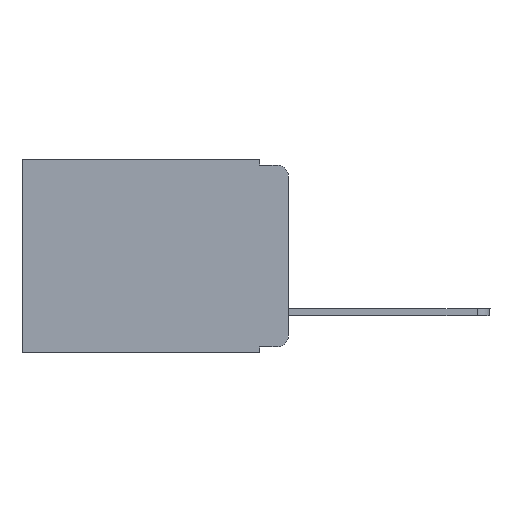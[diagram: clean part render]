
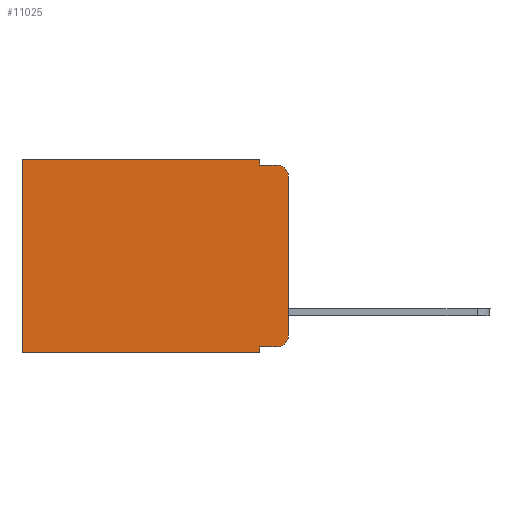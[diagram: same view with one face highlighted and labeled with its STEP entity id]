
A CAD part, left-side view. The second image highlights one B-rep face of the part: STEP entity #11025.
In plain terms, the highlighted planar face has unit normal (-1, 0, 0).
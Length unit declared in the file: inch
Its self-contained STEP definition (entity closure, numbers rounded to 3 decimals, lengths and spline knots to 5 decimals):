
#78 = VECTOR ( 'NONE', #16778, 39.37008 ) ;
#1495 = EDGE_CURVE ( 'NONE', #12598, #10663, #1684, .T. ) ;
#1622 = CARTESIAN_POINT ( 'NONE',  ( 0.298, 0.051, -0.333 ) ) ;
#1684 = LINE ( 'NONE', #5780, #8109 ) ;
#1957 = CARTESIAN_POINT ( 'NONE',  ( 0.298, 0.473, -0.343 ) ) ;
#2248 = CARTESIAN_POINT ( 'NONE',  ( 0.298, 0.051, 0. ) ) ;
#2581 = VERTEX_POINT ( 'NONE', #6371 ) ;
#3566 = VECTOR ( 'NONE', #10456, 39.37008 ) ;
#4105 = VERTEX_POINT ( 'NONE', #14018 ) ;
#4929 = ORIENTED_EDGE ( 'NONE', *, *, #22151, .F. ) ;
#5204 = ORIENTED_EDGE ( 'NONE', *, *, #13808, .T. ) ;
#5206 = CARTESIAN_POINT ( 'NONE',  ( 0.298, 0.02, -0.333 ) ) ;
#5630 = CARTESIAN_POINT ( 'NONE',  ( 0.298, 0., 0. ) ) ;
#5780 = CARTESIAN_POINT ( 'NONE',  ( 0.298, 0.051, -0.01 ) ) ;
#6371 = CARTESIAN_POINT ( 'NONE',  ( 0.298, 0.473, 0. ) ) ;
#6664 = VECTOR ( 'NONE', #14438, 39.37008 ) ;
#7050 = VERTEX_POINT ( 'NONE', #1957 ) ;
#7053 = DIRECTION ( 'NONE',  ( 0., 0., -1. ) ) ;
#7216 = DIRECTION ( 'NONE',  ( 1., 0., 0. ) ) ;
#7571 = PLANE ( 'NONE',  #8769 ) ;
#8033 = VERTEX_POINT ( 'NONE', #2248 ) ;
#8109 = VECTOR ( 'NONE', #9442, 39.37008 ) ;
#8580 = VECTOR ( 'NONE', #11817, 39.37008 ) ;
#8769 = AXIS2_PLACEMENT_3D ( 'NONE', #5630, #7216, #14965 ) ;
#8856 = CARTESIAN_POINT ( 'NONE',  ( 0.298, 0.02, -0.01 ) ) ;
#8882 = CARTESIAN_POINT ( 'NONE',  ( 0.298, 0.02, -0.03 ) ) ;
#9099 = DIRECTION ( 'NONE',  ( 0., 0., -1. ) ) ;
#9442 = DIRECTION ( 'NONE',  ( 0., -1., 0. ) ) ;
#9469 = EDGE_CURVE ( 'NONE', #20974, #21057, #21058, .T. ) ;
#10104 = ORIENTED_EDGE ( 'NONE', *, *, #12960, .T. ) ;
#10155 = CARTESIAN_POINT ( 'NONE',  ( 0.298, 0.051, -0.01 ) ) ;
#10189 = ORIENTED_EDGE ( 'NONE', *, *, #9469, .F. ) ;
#10456 = DIRECTION ( 'NONE',  ( 0., 1., 0. ) ) ;
#10519 = ORIENTED_EDGE ( 'NONE', *, *, #22406, .T. ) ;
#10549 = DIRECTION ( 'NONE',  ( -1., 0., 0. ) ) ;
#10663 = VERTEX_POINT ( 'NONE', #8856 ) ;
#10664 = DIRECTION ( 'NONE',  ( 0., 0., -1. ) ) ;
#11025 = ADVANCED_FACE ( 'NONE', ( #23717 ), #7571, .F. ) ;
#11306 = DIRECTION ( 'NONE',  ( 0., -1., 0. ) ) ;
#11679 = AXIS2_PLACEMENT_3D ( 'NONE', #8882, #23673, #7053 ) ;
#11817 = DIRECTION ( 'NONE',  ( 0., 0., -1. ) ) ;
#12023 = CARTESIAN_POINT ( 'NONE',  ( 0.298, 0., 0. ) ) ;
#12478 = CARTESIAN_POINT ( 'NONE',  ( 0.298, 0.02, -0.313 ) ) ;
#12598 = VERTEX_POINT ( 'NONE', #10155 ) ;
#12960 = EDGE_CURVE ( 'NONE', #8033, #2581, #17962, .T. ) ;
#13098 = EDGE_CURVE ( 'NONE', #8033, #12598, #20160, .T. ) ;
#13201 = EDGE_CURVE ( 'NONE', #4105, #7050, #15507, .T. ) ;
#13258 = CARTESIAN_POINT ( 'NONE',  ( 0.298, 0.051, 0. ) ) ;
#13263 = VECTOR ( 'NONE', #20746, 39.37008 ) ;
#13361 = CARTESIAN_POINT ( 'NONE',  ( 0.298, 0., -0.313 ) ) ;
#13689 = CARTESIAN_POINT ( 'NONE',  ( 0.298, 0., -0.343 ) ) ;
#13808 = EDGE_CURVE ( 'NONE', #2581, #7050, #14287, .T. ) ;
#13849 = EDGE_CURVE ( 'NONE', #16396, #21057, #18260, .T. ) ;
#14018 = CARTESIAN_POINT ( 'NONE',  ( 0.298, 0.051, -0.343 ) ) ;
#14287 = LINE ( 'NONE', #23766, #17073 ) ;
#14382 = ORIENTED_EDGE ( 'NONE', *, *, #19597, .T. ) ;
#14438 = DIRECTION ( 'NONE',  ( 0., 0., -1. ) ) ;
#14871 = EDGE_LOOP ( 'NONE', ( #10189, #10519, #16386, #23104, #10104, #5204, #19058, #4929, #14382, #17614 ) ) ;
#14965 = DIRECTION ( 'NONE',  ( 0., 0., -1. ) ) ;
#15507 = LINE ( 'NONE', #13689, #13263 ) ;
#16386 = ORIENTED_EDGE ( 'NONE', *, *, #1495, .F. ) ;
#16396 = VERTEX_POINT ( 'NONE', #5206 ) ;
#16778 = DIRECTION ( 'NONE',  ( 0., 0., -1. ) ) ;
#17073 = VECTOR ( 'NONE', #9099, 39.37008 ) ;
#17614 = ORIENTED_EDGE ( 'NONE', *, *, #13849, .T. ) ;
#17962 = LINE ( 'NONE', #12023, #3566 ) ;
#18260 = CIRCLE ( 'NONE', #22906, 0.02 ) ;
#18359 = LINE ( 'NONE', #22355, #23362 ) ;
#19058 = ORIENTED_EDGE ( 'NONE', *, *, #13201, .F. ) ;
#19597 = EDGE_CURVE ( 'NONE', #19691, #16396, #18359, .T. ) ;
#19691 = VERTEX_POINT ( 'NONE', #1622 ) ;
#20069 = CARTESIAN_POINT ( 'NONE',  ( 0.298, 0., -0.03 ) ) ;
#20160 = LINE ( 'NONE', #20283, #6664 ) ;
#20283 = CARTESIAN_POINT ( 'NONE',  ( 0.298, 0.051, 0. ) ) ;
#20617 = CIRCLE ( 'NONE', #11679, 0.02 ) ;
#20746 = DIRECTION ( 'NONE',  ( 0., 1., 0. ) ) ;
#20974 = VERTEX_POINT ( 'NONE', #20069 ) ;
#21057 = VERTEX_POINT ( 'NONE', #13361 ) ;
#21058 = LINE ( 'NONE', #21176, #8580 ) ;
#21176 = CARTESIAN_POINT ( 'NONE',  ( 0.298, 0., 0. ) ) ;
#22142 = LINE ( 'NONE', #13258, #78 ) ;
#22151 = EDGE_CURVE ( 'NONE', #19691, #4105, #22142, .T. ) ;
#22355 = CARTESIAN_POINT ( 'NONE',  ( 0.298, 0.051, -0.333 ) ) ;
#22406 = EDGE_CURVE ( 'NONE', #20974, #10663, #20617, .T. ) ;
#22906 = AXIS2_PLACEMENT_3D ( 'NONE', #12478, #10549, #10664 ) ;
#23104 = ORIENTED_EDGE ( 'NONE', *, *, #13098, .F. ) ;
#23362 = VECTOR ( 'NONE', #11306, 39.37008 ) ;
#23673 = DIRECTION ( 'NONE',  ( -1., 0., 0. ) ) ;
#23717 = FACE_OUTER_BOUND ( 'NONE', #14871, .T. ) ;
#23766 = CARTESIAN_POINT ( 'NONE',  ( 0.298, 0.473, 0. ) ) ;
